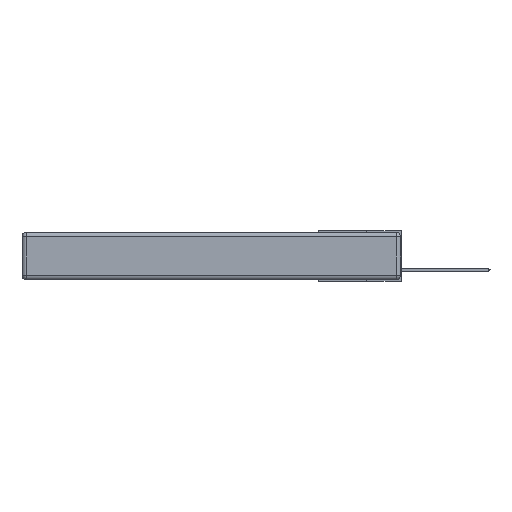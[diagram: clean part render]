
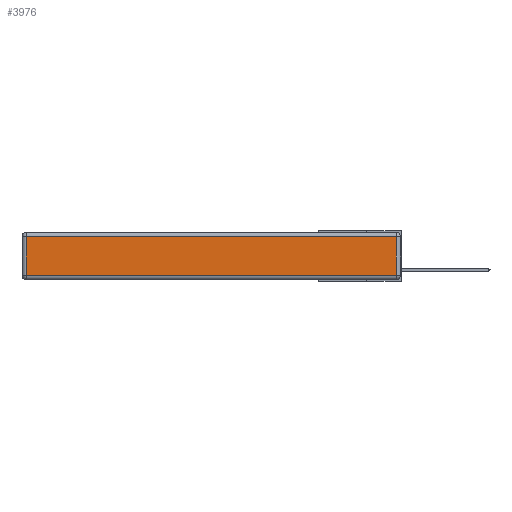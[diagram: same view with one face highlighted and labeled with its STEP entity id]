
A CAD part, left-side view. The second image highlights one B-rep face of the part: STEP entity #3976.
In plain terms, the highlighted planar face has unit normal (-1, 0, 0).
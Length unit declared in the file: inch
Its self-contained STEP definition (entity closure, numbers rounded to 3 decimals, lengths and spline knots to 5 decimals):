
#545 = DIRECTION ( 'NONE',  ( 0., -1., 0. ) ) ;
#1562 = CARTESIAN_POINT ( 'NONE',  ( 0., 0., -0.343 ) ) ;
#1918 = ORIENTED_EDGE ( 'NONE', *, *, #19142, .T. ) ;
#2535 = VERTEX_POINT ( 'NONE', #11004 ) ;
#2783 = FACE_OUTER_BOUND ( 'NONE', #7337, .T. ) ;
#3202 = VERTEX_POINT ( 'NONE', #5940 ) ;
#3976 = ADVANCED_FACE ( 'NONE', ( #2783 ), #10525, .T. ) ;
#4997 = CARTESIAN_POINT ( 'NONE',  ( 0., 2.75, -0.03 ) ) ;
#5073 = AXIS2_PLACEMENT_3D ( 'NONE', #1562, #15039, #12050 ) ;
#5255 = EDGE_CURVE ( 'NONE', #15408, #12112, #13650, .T. ) ;
#5940 = CARTESIAN_POINT ( 'NONE',  ( 0., 2.72, -0.313 ) ) ;
#6247 = VECTOR ( 'NONE', #545, 39.37008 ) ;
#6392 = VECTOR ( 'NONE', #9906, 39.37008 ) ;
#6437 = CARTESIAN_POINT ( 'NONE',  ( 0., 0., -0.313 ) ) ;
#7337 = EDGE_LOOP ( 'NONE', ( #7477, #1918, #8038, #13821 ) ) ;
#7477 = ORIENTED_EDGE ( 'NONE', *, *, #17621, .T. ) ;
#7949 = CARTESIAN_POINT ( 'NONE',  ( 0., 2.72, -0.03 ) ) ;
#8038 = ORIENTED_EDGE ( 'NONE', *, *, #5255, .T. ) ;
#8354 = LINE ( 'NONE', #6437, #6247 ) ;
#9186 = VECTOR ( 'NONE', #18208, 39.37008 ) ;
#9906 = DIRECTION ( 'NONE',  ( 0., 0., -1. ) ) ;
#9965 = LINE ( 'NONE', #19280, #11133 ) ;
#10525 = PLANE ( 'NONE',  #5073 ) ;
#11004 = CARTESIAN_POINT ( 'NONE',  ( 0., 0.03, -0.313 ) ) ;
#11133 = VECTOR ( 'NONE', #13443, 39.37008 ) ;
#11330 = LINE ( 'NONE', #17389, #6392 ) ;
#12050 = DIRECTION ( 'NONE',  ( 0., 0., 1. ) ) ;
#12112 = VERTEX_POINT ( 'NONE', #7949 ) ;
#13398 = CARTESIAN_POINT ( 'NONE',  ( 0., 0.03, -0.03 ) ) ;
#13443 = DIRECTION ( 'NONE',  ( 0., 0., 1. ) ) ;
#13650 = LINE ( 'NONE', #4997, #9186 ) ;
#13821 = ORIENTED_EDGE ( 'NONE', *, *, #15709, .T. ) ;
#15039 = DIRECTION ( 'NONE',  ( -1., 0., 0. ) ) ;
#15408 = VERTEX_POINT ( 'NONE', #13398 ) ;
#15709 = EDGE_CURVE ( 'NONE', #12112, #3202, #11330, .T. ) ;
#17389 = CARTESIAN_POINT ( 'NONE',  ( 0., 2.72, -0.343 ) ) ;
#17621 = EDGE_CURVE ( 'NONE', #3202, #2535, #8354, .T. ) ;
#18208 = DIRECTION ( 'NONE',  ( 0., 1., 0. ) ) ;
#19142 = EDGE_CURVE ( 'NONE', #2535, #15408, #9965, .T. ) ;
#19280 = CARTESIAN_POINT ( 'NONE',  ( 0., 0.03, -0.343 ) ) ;
